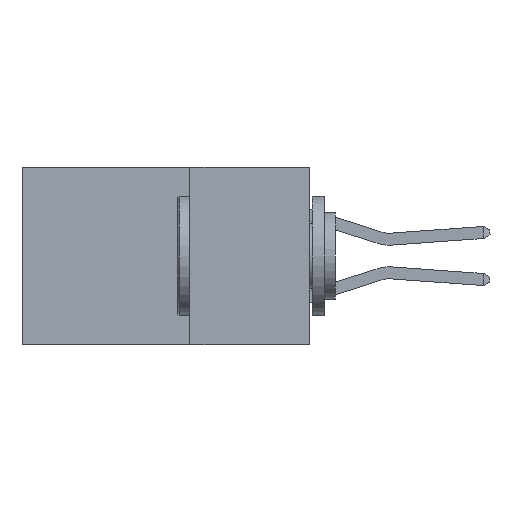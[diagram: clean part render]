
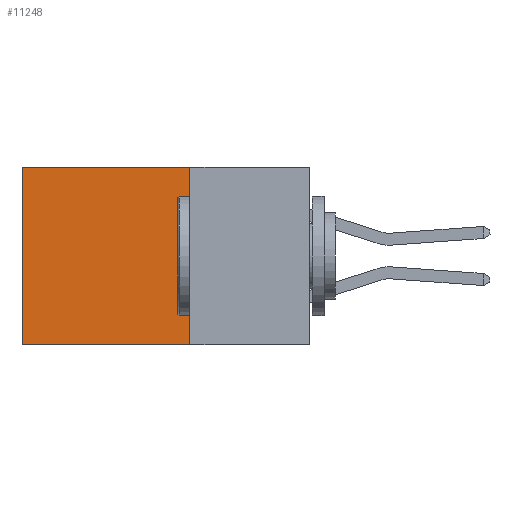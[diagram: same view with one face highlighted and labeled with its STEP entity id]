
A CAD part, left-side view. The second image highlights one B-rep face of the part: STEP entity #11248.
In plain terms, the highlighted planar face has unit normal (-1, 0, 0).
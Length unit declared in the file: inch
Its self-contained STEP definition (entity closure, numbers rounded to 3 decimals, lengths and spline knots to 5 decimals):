
#1330 = ORIENTED_EDGE ( 'NONE', *, *, #12150, .T. ) ;
#1623 = VERTEX_POINT ( 'NONE', #14355 ) ;
#2041 = DIRECTION ( 'NONE',  ( 0., 0., -1. ) ) ;
#2363 = VERTEX_POINT ( 'NONE', #9335 ) ;
#2869 = CARTESIAN_POINT ( 'NONE',  ( 0.298, 0.25, -0.37 ) ) ;
#3318 = CARTESIAN_POINT ( 'NONE',  ( 0.298, 0.25, 0. ) ) ;
#3361 = DIRECTION ( 'NONE',  ( 0., 0., -1. ) ) ;
#3413 = AXIS2_PLACEMENT_3D ( 'NONE', #7872, #9063, #2041 ) ;
#4545 = ORIENTED_EDGE ( 'NONE', *, *, #5037, .T. ) ;
#5037 = EDGE_CURVE ( 'NONE', #7279, #11099, #12699, .T. ) ;
#5243 = FACE_OUTER_BOUND ( 'NONE', #11842, .T. ) ;
#5748 = CARTESIAN_POINT ( 'NONE',  ( 0.298, 0.6, 0. ) ) ;
#6647 = LINE ( 'NONE', #5748, #9753 ) ;
#6959 = LINE ( 'NONE', #11488, #10746 ) ;
#7279 = VERTEX_POINT ( 'NONE', #9533 ) ;
#7872 = CARTESIAN_POINT ( 'NONE',  ( 0.298, 0.25, 0. ) ) ;
#9002 = EDGE_CURVE ( 'NONE', #7279, #1623, #6959, .T. ) ;
#9063 = DIRECTION ( 'NONE',  ( 1., 0., 0. ) ) ;
#9153 = LINE ( 'NONE', #2869, #11879 ) ;
#9335 = CARTESIAN_POINT ( 'NONE',  ( 0.298, 0.6, -0.37 ) ) ;
#9533 = CARTESIAN_POINT ( 'NONE',  ( 0.298, 0.25, 0. ) ) ;
#9753 = VECTOR ( 'NONE', #3361, 39.37008 ) ;
#9871 = DIRECTION ( 'NONE',  ( 0., 1., 0. ) ) ;
#10714 = ORIENTED_EDGE ( 'NONE', *, *, #13803, .F. ) ;
#10746 = VECTOR ( 'NONE', #13836, 39.37008 ) ;
#11048 = CARTESIAN_POINT ( 'NONE',  ( 0.298, 0.6, 0. ) ) ;
#11099 = VERTEX_POINT ( 'NONE', #11048 ) ;
#11248 = ADVANCED_FACE ( 'NONE', ( #5243 ), #14850, .F. ) ;
#11488 = CARTESIAN_POINT ( 'NONE',  ( 0.298, 0.25, 0. ) ) ;
#11842 = EDGE_LOOP ( 'NONE', ( #1330, #10714, #14894, #4545 ) ) ;
#11879 = VECTOR ( 'NONE', #9871, 39.37008 ) ;
#12150 = EDGE_CURVE ( 'NONE', #11099, #2363, #6647, .T. ) ;
#12331 = VECTOR ( 'NONE', #12726, 39.37008 ) ;
#12699 = LINE ( 'NONE', #3318, #12331 ) ;
#12726 = DIRECTION ( 'NONE',  ( 0., 1., 0. ) ) ;
#13803 = EDGE_CURVE ( 'NONE', #1623, #2363, #9153, .T. ) ;
#13836 = DIRECTION ( 'NONE',  ( 0., 0., -1. ) ) ;
#14355 = CARTESIAN_POINT ( 'NONE',  ( 0.298, 0.25, -0.37 ) ) ;
#14850 = PLANE ( 'NONE',  #3413 ) ;
#14894 = ORIENTED_EDGE ( 'NONE', *, *, #9002, .F. ) ;
